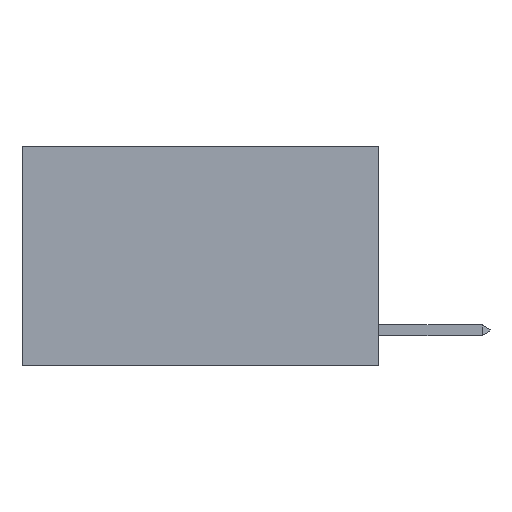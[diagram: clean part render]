
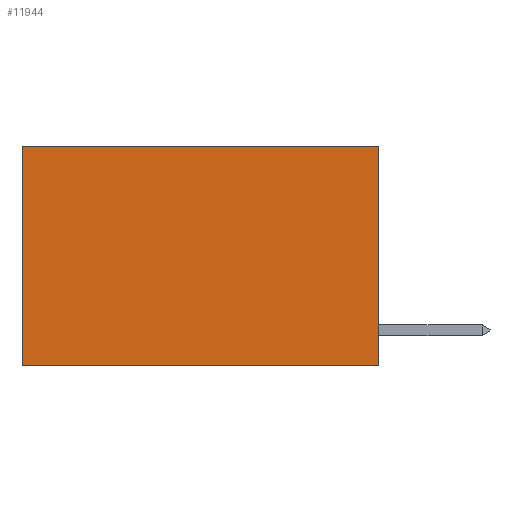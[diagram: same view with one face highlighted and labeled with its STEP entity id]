
A CAD part, left-side view. The second image highlights one B-rep face of the part: STEP entity #11944.
In plain terms, the highlighted planar face has unit normal (-1, 0, 0).
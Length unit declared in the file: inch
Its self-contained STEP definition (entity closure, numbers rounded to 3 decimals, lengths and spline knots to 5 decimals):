
#364 = DIRECTION ( 'NONE',  ( 0., 0., -1. ) ) ;
#451 = ORIENTED_EDGE ( 'NONE', *, *, #6296, .F. ) ;
#661 = ORIENTED_EDGE ( 'NONE', *, *, #13672, .F. ) ;
#1317 = VECTOR ( 'NONE', #9992, 39.37008 ) ;
#1437 = PLANE ( 'NONE',  #8106 ) ;
#1528 = LINE ( 'NONE', #11972, #1317 ) ;
#1926 = EDGE_LOOP ( 'NONE', ( #3782, #451, #661, #2798 ) ) ;
#1971 = VECTOR ( 'NONE', #364, 39.37008 ) ;
#2364 = CARTESIAN_POINT ( 'NONE',  ( 0.2625, 0.6, -0.37 ) ) ;
#2798 = ORIENTED_EDGE ( 'NONE', *, *, #4294, .T. ) ;
#3238 = CARTESIAN_POINT ( 'NONE',  ( 0.2625, 0.6, 0. ) ) ;
#3782 = ORIENTED_EDGE ( 'NONE', *, *, #6266, .T. ) ;
#3943 = VECTOR ( 'NONE', #7682, 39.37008 ) ;
#4294 = EDGE_CURVE ( 'NONE', #10761, #13105, #1528, .T. ) ;
#4599 = VECTOR ( 'NONE', #6739, 39.37008 ) ;
#5534 = CARTESIAN_POINT ( 'NONE',  ( 0.2625, 0., -0.37 ) ) ;
#5892 = VERTEX_POINT ( 'NONE', #11249 ) ;
#6266 = EDGE_CURVE ( 'NONE', #13105, #10925, #9875, .T. ) ;
#6296 = EDGE_CURVE ( 'NONE', #5892, #10925, #8652, .T. ) ;
#6739 = DIRECTION ( 'NONE',  ( 0., 0., -1. ) ) ;
#7682 = DIRECTION ( 'NONE',  ( 0., 1., 0. ) ) ;
#8106 = AXIS2_PLACEMENT_3D ( 'NONE', #8890, #9882, #13191 ) ;
#8652 = LINE ( 'NONE', #5534, #3943 ) ;
#8890 = CARTESIAN_POINT ( 'NONE',  ( 0.2625, 0., 0. ) ) ;
#9875 = LINE ( 'NONE', #12060, #4599 ) ;
#9882 = DIRECTION ( 'NONE',  ( 1., 0., 0. ) ) ;
#9992 = DIRECTION ( 'NONE',  ( 0., 1., 0. ) ) ;
#10761 = VERTEX_POINT ( 'NONE', #13654 ) ;
#10925 = VERTEX_POINT ( 'NONE', #2364 ) ;
#10947 = FACE_OUTER_BOUND ( 'NONE', #1926, .T. ) ;
#11249 = CARTESIAN_POINT ( 'NONE',  ( 0.2625, 0., -0.37 ) ) ;
#11944 = ADVANCED_FACE ( 'NONE', ( #10947 ), #1437, .F. ) ;
#11972 = CARTESIAN_POINT ( 'NONE',  ( 0.2625, 0., 0. ) ) ;
#12059 = LINE ( 'NONE', #12118, #1971 ) ;
#12060 = CARTESIAN_POINT ( 'NONE',  ( 0.2625, 0.6, 0. ) ) ;
#12118 = CARTESIAN_POINT ( 'NONE',  ( 0.2625, 0., 0. ) ) ;
#13105 = VERTEX_POINT ( 'NONE', #3238 ) ;
#13191 = DIRECTION ( 'NONE',  ( 0., 0., -1. ) ) ;
#13654 = CARTESIAN_POINT ( 'NONE',  ( 0.2625, 0., 0. ) ) ;
#13672 = EDGE_CURVE ( 'NONE', #10761, #5892, #12059, .T. ) ;
